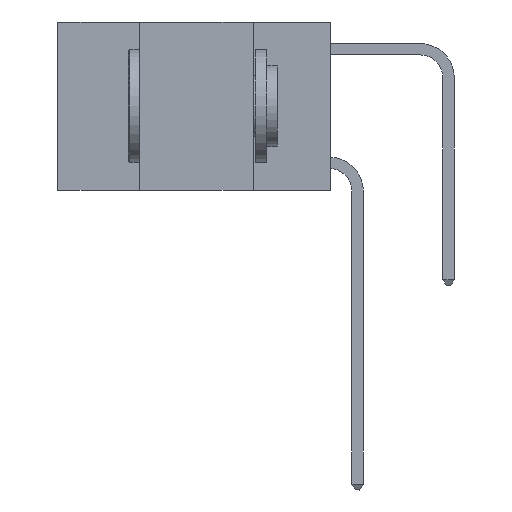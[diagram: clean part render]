
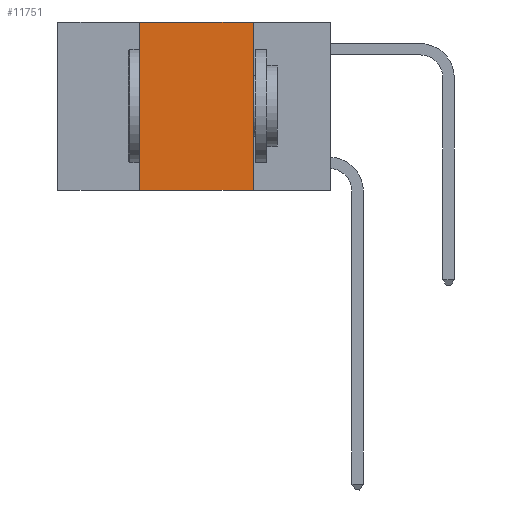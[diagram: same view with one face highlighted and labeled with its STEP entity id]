
A CAD part, left-side view. The second image highlights one B-rep face of the part: STEP entity #11751.
In plain terms, the highlighted planar face has unit normal (-1, 0, 0).
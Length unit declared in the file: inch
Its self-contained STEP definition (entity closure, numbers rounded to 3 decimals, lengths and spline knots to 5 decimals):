
#370 = DIRECTION ( 'NONE',  ( 0., 0., 1. ) ) ;
#643 = LINE ( 'NONE', #12297, #19531 ) ;
#692 = LINE ( 'NONE', #15647, #6893 ) ;
#1030 = CARTESIAN_POINT ( 'NONE',  ( 0., 0.17, 0. ) ) ;
#1482 = VERTEX_POINT ( 'NONE', #17689 ) ;
#1865 = CARTESIAN_POINT ( 'NONE',  ( 0., 0.17, -0.37 ) ) ;
#2117 = ORIENTED_EDGE ( 'NONE', *, *, #14414, .T. ) ;
#2867 = VERTEX_POINT ( 'NONE', #1030 ) ;
#3536 = CARTESIAN_POINT ( 'NONE',  ( 0., 0.6, -0.37 ) ) ;
#3952 = CARTESIAN_POINT ( 'NONE',  ( 0., 0.6, 0. ) ) ;
#6066 = ORIENTED_EDGE ( 'NONE', *, *, #12810, .F. ) ;
#6893 = VECTOR ( 'NONE', #8609, 39.37008 ) ;
#8609 = DIRECTION ( 'NONE',  ( 0., 0., -1. ) ) ;
#9886 = ORIENTED_EDGE ( 'NONE', *, *, #11522, .F. ) ;
#10727 = DIRECTION ( 'NONE',  ( 0., -1., 0. ) ) ;
#11284 = LINE ( 'NONE', #3536, #15008 ) ;
#11522 = EDGE_CURVE ( 'NONE', #2867, #22072, #692, .T. ) ;
#11751 = ADVANCED_FACE ( 'NONE', ( #21810 ), #22178, .F. ) ;
#12188 = LINE ( 'NONE', #18335, #22079 ) ;
#12297 = CARTESIAN_POINT ( 'NONE',  ( 0., 0.6, 0. ) ) ;
#12358 = EDGE_CURVE ( 'NONE', #13874, #1482, #12188, .T. ) ;
#12810 = EDGE_CURVE ( 'NONE', #1482, #2867, #643, .T. ) ;
#13292 = ORIENTED_EDGE ( 'NONE', *, *, #12358, .F. ) ;
#13874 = VERTEX_POINT ( 'NONE', #16494 ) ;
#14414 = EDGE_CURVE ( 'NONE', #13874, #22072, #11284, .T. ) ;
#15008 = VECTOR ( 'NONE', #10727, 39.37008 ) ;
#15647 = CARTESIAN_POINT ( 'NONE',  ( 0., 0.17, 0. ) ) ;
#16013 = AXIS2_PLACEMENT_3D ( 'NONE', #3952, #20371, #18441 ) ;
#16051 = DIRECTION ( 'NONE',  ( 0., -1., 0. ) ) ;
#16494 = CARTESIAN_POINT ( 'NONE',  ( 0., 0.42, -0.37 ) ) ;
#17689 = CARTESIAN_POINT ( 'NONE',  ( 0., 0.42, 0. ) ) ;
#18335 = CARTESIAN_POINT ( 'NONE',  ( 0., 0.42, 0. ) ) ;
#18441 = DIRECTION ( 'NONE',  ( 0., 0., -1. ) ) ;
#19531 = VECTOR ( 'NONE', #16051, 39.37008 ) ;
#20371 = DIRECTION ( 'NONE',  ( 1., 0., 0. ) ) ;
#21810 = FACE_OUTER_BOUND ( 'NONE', #22973, .T. ) ;
#22072 = VERTEX_POINT ( 'NONE', #1865 ) ;
#22079 = VECTOR ( 'NONE', #370, 39.37008 ) ;
#22178 = PLANE ( 'NONE',  #16013 ) ;
#22973 = EDGE_LOOP ( 'NONE', ( #9886, #6066, #13292, #2117 ) ) ;
